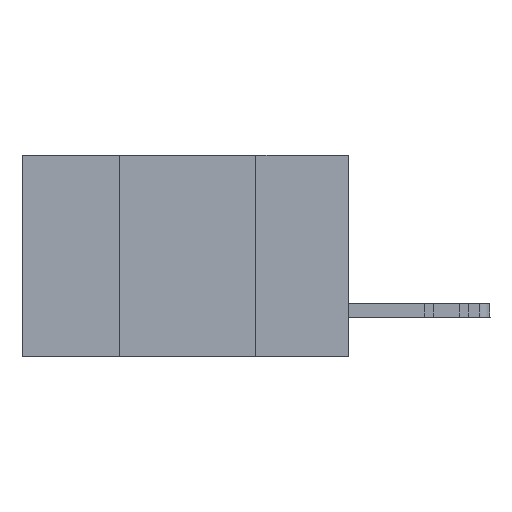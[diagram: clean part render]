
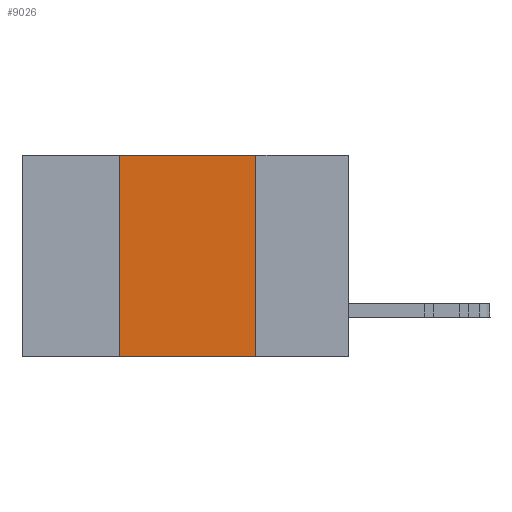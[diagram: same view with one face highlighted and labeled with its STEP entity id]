
A CAD part, left-side view. The second image highlights one B-rep face of the part: STEP entity #9026.
In plain terms, the highlighted planar face has unit normal (-1, 0, 0).
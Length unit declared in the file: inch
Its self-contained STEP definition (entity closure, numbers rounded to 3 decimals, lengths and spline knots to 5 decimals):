
#1207 = VERTEX_POINT ( 'NONE', #18957 ) ;
#2956 = ORIENTED_EDGE ( 'NONE', *, *, #24055, .F. ) ;
#3139 = CARTESIAN_POINT ( 'NONE',  ( 0., 0.42, 0. ) ) ;
#4324 = FACE_OUTER_BOUND ( 'NONE', #15375, .T. ) ;
#4868 = VECTOR ( 'NONE', #23414, 39.37008 ) ;
#7272 = VECTOR ( 'NONE', #9672, 39.37008 ) ;
#8647 = CARTESIAN_POINT ( 'NONE',  ( 0., 0.17, 0. ) ) ;
#8958 = DIRECTION ( 'NONE',  ( 1., 0., 0. ) ) ;
#9026 = ADVANCED_FACE ( 'NONE', ( #4324 ), #23008, .F. ) ;
#9672 = DIRECTION ( 'NONE',  ( 0., -1., 0. ) ) ;
#11171 = LINE ( 'NONE', #8647, #4868 ) ;
#11324 = ORIENTED_EDGE ( 'NONE', *, *, #17226, .F. ) ;
#12818 = VECTOR ( 'NONE', #23655, 39.37008 ) ;
#15375 = EDGE_LOOP ( 'NONE', ( #20691, #11324, #2956, #25680 ) ) ;
#16147 = LINE ( 'NONE', #19099, #12818 ) ;
#16232 = VERTEX_POINT ( 'NONE', #3139 ) ;
#17226 = EDGE_CURVE ( 'NONE', #16232, #26603, #16147, .T. ) ;
#18773 = AXIS2_PLACEMENT_3D ( 'NONE', #29945, #8958, #18868 ) ;
#18868 = DIRECTION ( 'NONE',  ( 0., 0., -1. ) ) ;
#18957 = CARTESIAN_POINT ( 'NONE',  ( 0., 0.42, -0.37 ) ) ;
#19026 = EDGE_CURVE ( 'NONE', #26603, #28368, #11171, .T. ) ;
#19099 = CARTESIAN_POINT ( 'NONE',  ( 0., 0.6, 0. ) ) ;
#19200 = VECTOR ( 'NONE', #26181, 39.37008 ) ;
#20691 = ORIENTED_EDGE ( 'NONE', *, *, #19026, .F. ) ;
#20730 = CARTESIAN_POINT ( 'NONE',  ( 0., 0.17, -0.37 ) ) ;
#21349 = CARTESIAN_POINT ( 'NONE',  ( 0., 0.42, 0. ) ) ;
#22226 = EDGE_CURVE ( 'NONE', #1207, #28368, #26194, .T. ) ;
#23008 = PLANE ( 'NONE',  #18773 ) ;
#23414 = DIRECTION ( 'NONE',  ( 0., 0., -1. ) ) ;
#23655 = DIRECTION ( 'NONE',  ( 0., -1., 0. ) ) ;
#24055 = EDGE_CURVE ( 'NONE', #1207, #16232, #25483, .T. ) ;
#25483 = LINE ( 'NONE', #21349, #19200 ) ;
#25680 = ORIENTED_EDGE ( 'NONE', *, *, #22226, .T. ) ;
#26181 = DIRECTION ( 'NONE',  ( 0., 0., 1. ) ) ;
#26194 = LINE ( 'NONE', #29003, #7272 ) ;
#26603 = VERTEX_POINT ( 'NONE', #27313 ) ;
#27313 = CARTESIAN_POINT ( 'NONE',  ( 0., 0.17, 0. ) ) ;
#28368 = VERTEX_POINT ( 'NONE', #20730 ) ;
#29003 = CARTESIAN_POINT ( 'NONE',  ( 0., 0.6, -0.37 ) ) ;
#29945 = CARTESIAN_POINT ( 'NONE',  ( 0., 0.6, 0. ) ) ;
